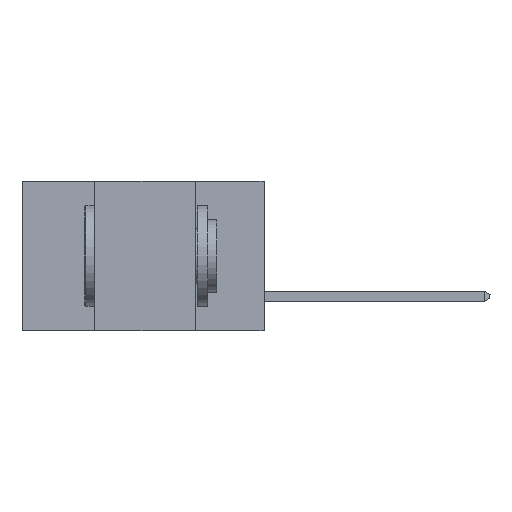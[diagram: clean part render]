
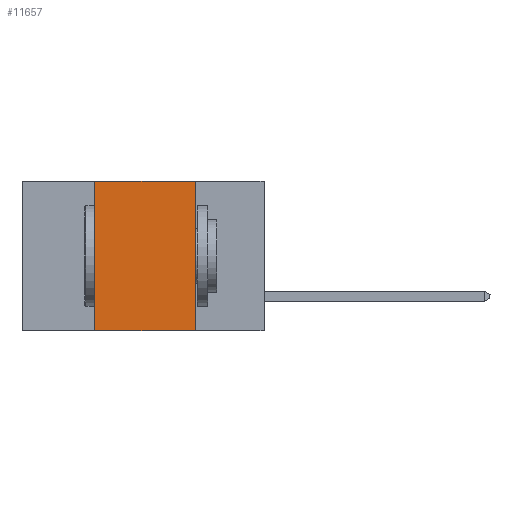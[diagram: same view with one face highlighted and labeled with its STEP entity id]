
A CAD part, left-side view. The second image highlights one B-rep face of the part: STEP entity #11657.
In plain terms, the highlighted planar face has unit normal (-1, 0, 0).
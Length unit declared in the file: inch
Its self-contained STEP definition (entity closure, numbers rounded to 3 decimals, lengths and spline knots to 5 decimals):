
#66 = ORIENTED_EDGE ( 'NONE', *, *, #6068, .F. ) ;
#745 = VERTEX_POINT ( 'NONE', #1488 ) ;
#1244 = LINE ( 'NONE', #12429, #12125 ) ;
#1331 = DIRECTION ( 'NONE',  ( 0., 0., 1. ) ) ;
#1423 = DIRECTION ( 'NONE',  ( 0., 0., -1. ) ) ;
#1488 = CARTESIAN_POINT ( 'NONE',  ( 0., 0.17, -0.37 ) ) ;
#1495 = DIRECTION ( 'NONE',  ( 1., 0., 0. ) ) ;
#2137 = CARTESIAN_POINT ( 'NONE',  ( 0., 0.42, -0.37 ) ) ;
#2143 = DIRECTION ( 'NONE',  ( 0., -1., 0. ) ) ;
#2234 = EDGE_CURVE ( 'NONE', #13555, #14405, #2363, .T. ) ;
#2363 = LINE ( 'NONE', #6849, #9402 ) ;
#2528 = CARTESIAN_POINT ( 'NONE',  ( 0., 0.42, -0.37 ) ) ;
#2540 = CARTESIAN_POINT ( 'NONE',  ( 0., 0.6, 0. ) ) ;
#3646 = CARTESIAN_POINT ( 'NONE',  ( 0., 0.6, -0.37 ) ) ;
#3702 = PLANE ( 'NONE',  #13796 ) ;
#3939 = EDGE_LOOP ( 'NONE', ( #9328, #12110, #66, #14130 ) ) ;
#4785 = DIRECTION ( 'NONE',  ( 0., 0., -1. ) ) ;
#5637 = EDGE_CURVE ( 'NONE', #8256, #745, #13784, .T. ) ;
#6068 = EDGE_CURVE ( 'NONE', #8256, #13555, #8090, .T. ) ;
#6354 = CARTESIAN_POINT ( 'NONE',  ( 0., 0.17, 0. ) ) ;
#6492 = VECTOR ( 'NONE', #12469, 39.37008 ) ;
#6849 = CARTESIAN_POINT ( 'NONE',  ( 0., 0.6, 0. ) ) ;
#8090 = LINE ( 'NONE', #2528, #14181 ) ;
#8256 = VERTEX_POINT ( 'NONE', #2137 ) ;
#9328 = ORIENTED_EDGE ( 'NONE', *, *, #10697, .F. ) ;
#9402 = VECTOR ( 'NONE', #2143, 39.37008 ) ;
#10697 = EDGE_CURVE ( 'NONE', #14405, #745, #1244, .T. ) ;
#11551 = CARTESIAN_POINT ( 'NONE',  ( 0., 0.42, 0. ) ) ;
#11657 = ADVANCED_FACE ( 'NONE', ( #12674 ), #3702, .F. ) ;
#12110 = ORIENTED_EDGE ( 'NONE', *, *, #2234, .F. ) ;
#12125 = VECTOR ( 'NONE', #4785, 39.37008 ) ;
#12429 = CARTESIAN_POINT ( 'NONE',  ( 0., 0.17, -0.37 ) ) ;
#12469 = DIRECTION ( 'NONE',  ( 0., -1., 0. ) ) ;
#12674 = FACE_OUTER_BOUND ( 'NONE', #3939, .T. ) ;
#13555 = VERTEX_POINT ( 'NONE', #11551 ) ;
#13784 = LINE ( 'NONE', #3646, #6492 ) ;
#13796 = AXIS2_PLACEMENT_3D ( 'NONE', #2540, #1495, #1423 ) ;
#14130 = ORIENTED_EDGE ( 'NONE', *, *, #5637, .T. ) ;
#14181 = VECTOR ( 'NONE', #1331, 39.37008 ) ;
#14405 = VERTEX_POINT ( 'NONE', #6354 ) ;
